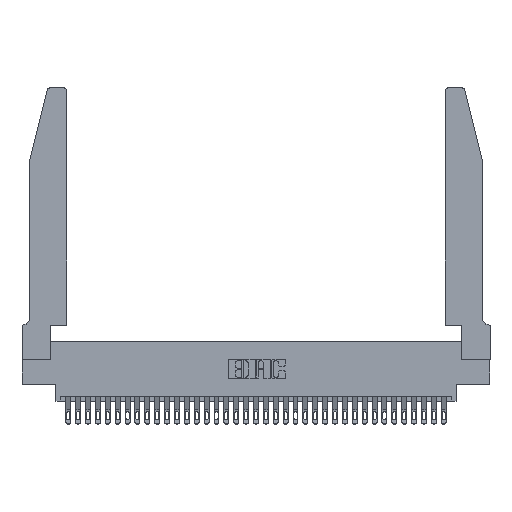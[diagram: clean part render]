
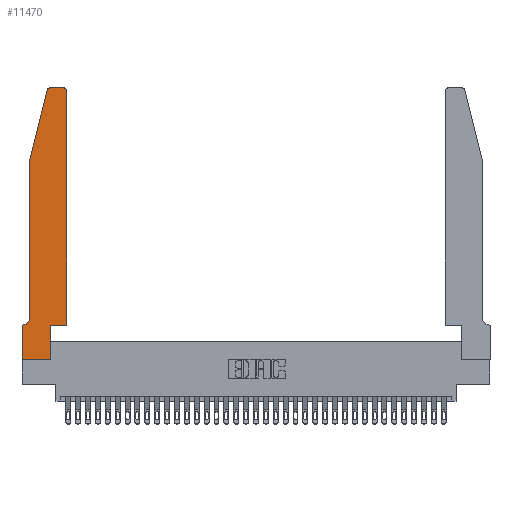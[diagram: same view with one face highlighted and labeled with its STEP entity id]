
A CAD part, top view. The second image highlights one B-rep face of the part: STEP entity #11470.
In plain terms, the highlighted planar face has unit normal (0, 0, 1).
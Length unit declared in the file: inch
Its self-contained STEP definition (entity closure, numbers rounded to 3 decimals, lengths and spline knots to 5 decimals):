
#70 = ORIENTED_EDGE ( 'NONE', *, *, #12679, .T. ) ;
#560 = CARTESIAN_POINT ( 'NONE',  ( 0.0755, 2., 0.37 ) ) ;
#1693 = ORIENTED_EDGE ( 'NONE', *, *, #9112, .T. ) ;
#1797 = DIRECTION ( 'NONE',  ( 0., 0., -1. ) ) ;
#2720 = ORIENTED_EDGE ( 'NONE', *, *, #35310, .T. ) ;
#2890 = CARTESIAN_POINT ( 'NONE',  ( 0.0755, 0.42, 0.37 ) ) ;
#3278 = LINE ( 'NONE', #18330, #29558 ) ;
#4439 = CARTESIAN_POINT ( 'NONE',  ( 0.0755, 0.35, 0.37 ) ) ;
#5083 = DIRECTION ( 'NONE',  ( -1., 0., 0. ) ) ;
#5175 = VECTOR ( 'NONE', #27840, 39.37008 ) ;
#5622 = LINE ( 'NONE', #18789, #19276 ) ;
#5840 = LINE ( 'NONE', #4439, #32056 ) ;
#6165 = DIRECTION ( 'NONE',  ( 1., 0., 0. ) ) ;
#7711 = ORIENTED_EDGE ( 'NONE', *, *, #14329, .T. ) ;
#7730 = VERTEX_POINT ( 'NONE', #30343 ) ;
#7920 = CARTESIAN_POINT ( 'NONE',  ( 0.2865, 0., 0.37 ) ) ;
#8357 = CIRCLE ( 'NONE', #15004, 0.03 ) ;
#8495 = LINE ( 'NONE', #14490, #24272 ) ;
#8651 = VERTEX_POINT ( 'NONE', #2890 ) ;
#8947 = CIRCLE ( 'NONE', #25528, 0.07 ) ;
#9102 = CARTESIAN_POINT ( 'NONE',  ( 0.0755, 2., 0.37 ) ) ;
#9112 = EDGE_CURVE ( 'NONE', #30752, #10468, #8495, .T. ) ;
#9508 = LINE ( 'NONE', #15142, #5175 ) ;
#10468 = VERTEX_POINT ( 'NONE', #18739 ) ;
#10966 = VECTOR ( 'NONE', #33931, 39.37008 ) ;
#11053 = EDGE_CURVE ( 'NONE', #17450, #26091, #8357, .T. ) ;
#11327 = CARTESIAN_POINT ( 'NONE',  ( 0.25487, 2.72718, 0.37 ) ) ;
#11470 = ADVANCED_FACE ( 'NONE', ( #24537 ), #17871, .T. ) ;
#11527 = LINE ( 'NONE', #18308, #27795 ) ;
#12053 = EDGE_CURVE ( 'NONE', #13998, #17450, #5622, .T. ) ;
#12392 = CARTESIAN_POINT ( 'NONE',  ( 0.4205, 2.72, 0.37 ) ) ;
#12522 = DIRECTION ( 'NONE',  ( 1., 0., 0. ) ) ;
#12679 = EDGE_CURVE ( 'NONE', #17484, #19641, #15216, .T. ) ;
#12930 = DIRECTION ( 'NONE',  ( 0., 1., 0. ) ) ;
#13293 = EDGE_CURVE ( 'NONE', #26091, #25536, #9508, .T. ) ;
#13767 = ORIENTED_EDGE ( 'NONE', *, *, #12053, .T. ) ;
#13998 = VERTEX_POINT ( 'NONE', #27314 ) ;
#14329 = EDGE_CURVE ( 'NONE', #14795, #30752, #3278, .T. ) ;
#14490 = CARTESIAN_POINT ( 'NONE',  ( 0.4505, 0.35, 0.37 ) ) ;
#14795 = VERTEX_POINT ( 'NONE', #7920 ) ;
#15004 = AXIS2_PLACEMENT_3D ( 'NONE', #16599, #27986, #22019 ) ;
#15134 = CARTESIAN_POINT ( 'NONE',  ( 0.284, 2.75, 0.37 ) ) ;
#15142 = CARTESIAN_POINT ( 'NONE',  ( 0.0755, 2., 0.37 ) ) ;
#15216 = LINE ( 'NONE', #34812, #29221 ) ;
#15532 = CARTESIAN_POINT ( 'NONE',  ( 0.0055, 0.42, 0.37 ) ) ;
#16023 = CARTESIAN_POINT ( 'NONE',  ( 0., 0.35, 0.37 ) ) ;
#16104 = DIRECTION ( 'NONE',  ( 0., 1., 0. ) ) ;
#16599 = CARTESIAN_POINT ( 'NONE',  ( 0.284, 2.72, 0.37 ) ) ;
#16825 = ORIENTED_EDGE ( 'NONE', *, *, #20357, .T. ) ;
#17450 = VERTEX_POINT ( 'NONE', #15134 ) ;
#17484 = VERTEX_POINT ( 'NONE', #16023 ) ;
#17580 = AXIS2_PLACEMENT_3D ( 'NONE', #20244, #23805, #26843 ) ;
#17871 = PLANE ( 'NONE',  #17580 ) ;
#18308 = CARTESIAN_POINT ( 'NONE',  ( 0., 0., 0.37 ) ) ;
#18330 = CARTESIAN_POINT ( 'NONE',  ( 0.2865, 0.35, 0.37 ) ) ;
#18560 = LINE ( 'NONE', #24464, #27302 ) ;
#18739 = CARTESIAN_POINT ( 'NONE',  ( 0.4505, 0.35, 0.37 ) ) ;
#18789 = CARTESIAN_POINT ( 'NONE',  ( 0.2605, 2.75, 0.37 ) ) ;
#19276 = VECTOR ( 'NONE', #5083, 39.37008 ) ;
#19641 = VERTEX_POINT ( 'NONE', #31141 ) ;
#20244 = CARTESIAN_POINT ( 'NONE',  ( 0., 0.35, 0.37 ) ) ;
#20268 = CARTESIAN_POINT ( 'NONE',  ( 0.4505, 2.72, 0.37 ) ) ;
#20357 = EDGE_CURVE ( 'NONE', #22167, #13998, #34745, .T. ) ;
#21496 = DIRECTION ( 'NONE',  ( -1., 0., 0. ) ) ;
#21833 = ORIENTED_EDGE ( 'NONE', *, *, #35883, .T. ) ;
#22019 = DIRECTION ( 'NONE',  ( 1., 0., 0. ) ) ;
#22130 = EDGE_CURVE ( 'NONE', #19641, #14795, #11527, .T. ) ;
#22167 = VERTEX_POINT ( 'NONE', #20268 ) ;
#23738 = DIRECTION ( 'NONE',  ( 0., -1., 0. ) ) ;
#23805 = DIRECTION ( 'NONE',  ( 0., 0., 1. ) ) ;
#24272 = VECTOR ( 'NONE', #6165, 39.37008 ) ;
#24464 = CARTESIAN_POINT ( 'NONE',  ( 0.4505, 0.35, 0.37 ) ) ;
#24533 = DIRECTION ( 'NONE',  ( -1., 0., 0. ) ) ;
#24537 = FACE_OUTER_BOUND ( 'NONE', #28989, .T. ) ;
#25274 = ORIENTED_EDGE ( 'NONE', *, *, #13293, .T. ) ;
#25528 = AXIS2_PLACEMENT_3D ( 'NONE', #15532, #1797, #24533 ) ;
#25536 = VERTEX_POINT ( 'NONE', #560 ) ;
#25830 = LINE ( 'NONE', #9102, #10966 ) ;
#26091 = VERTEX_POINT ( 'NONE', #11327 ) ;
#26843 = DIRECTION ( 'NONE',  ( 1., 0., 0. ) ) ;
#27302 = VECTOR ( 'NONE', #16104, 39.37008 ) ;
#27314 = CARTESIAN_POINT ( 'NONE',  ( 0.4205, 2.75, 0.37 ) ) ;
#27720 = AXIS2_PLACEMENT_3D ( 'NONE', #12392, #34542, #12522 ) ;
#27795 = VECTOR ( 'NONE', #35428, 39.37008 ) ;
#27840 = DIRECTION ( 'NONE',  ( -0.239, -0.971, 0. ) ) ;
#27986 = DIRECTION ( 'NONE',  ( 0., 0., 1. ) ) ;
#28989 = EDGE_LOOP ( 'NONE', ( #13767, #36207, #25274, #33625, #2720, #21833, #70, #29751, #7711, #1693, #30853, #16825 ) ) ;
#29221 = VECTOR ( 'NONE', #23738, 39.37008 ) ;
#29558 = VECTOR ( 'NONE', #12930, 39.37008 ) ;
#29751 = ORIENTED_EDGE ( 'NONE', *, *, #22130, .T. ) ;
#30343 = CARTESIAN_POINT ( 'NONE',  ( 0.0055, 0.35, 0.37 ) ) ;
#30752 = VERTEX_POINT ( 'NONE', #30901 ) ;
#30853 = ORIENTED_EDGE ( 'NONE', *, *, #36006, .T. ) ;
#30901 = CARTESIAN_POINT ( 'NONE',  ( 0.2865, 0.35, 0.37 ) ) ;
#31141 = CARTESIAN_POINT ( 'NONE',  ( 0., 0., 0.37 ) ) ;
#32056 = VECTOR ( 'NONE', #21496, 39.37008 ) ;
#33625 = ORIENTED_EDGE ( 'NONE', *, *, #34431, .T. ) ;
#33931 = DIRECTION ( 'NONE',  ( 0., -1., 0. ) ) ;
#34431 = EDGE_CURVE ( 'NONE', #25536, #8651, #25830, .T. ) ;
#34542 = DIRECTION ( 'NONE',  ( 0., 0., 1. ) ) ;
#34745 = CIRCLE ( 'NONE', #27720, 0.03 ) ;
#34812 = CARTESIAN_POINT ( 'NONE',  ( 0., 0., 0.37 ) ) ;
#35310 = EDGE_CURVE ( 'NONE', #8651, #7730, #8947, .T. ) ;
#35428 = DIRECTION ( 'NONE',  ( 1., 0., 0. ) ) ;
#35883 = EDGE_CURVE ( 'NONE', #7730, #17484, #5840, .T. ) ;
#36006 = EDGE_CURVE ( 'NONE', #10468, #22167, #18560, .T. ) ;
#36207 = ORIENTED_EDGE ( 'NONE', *, *, #11053, .T. ) ;
